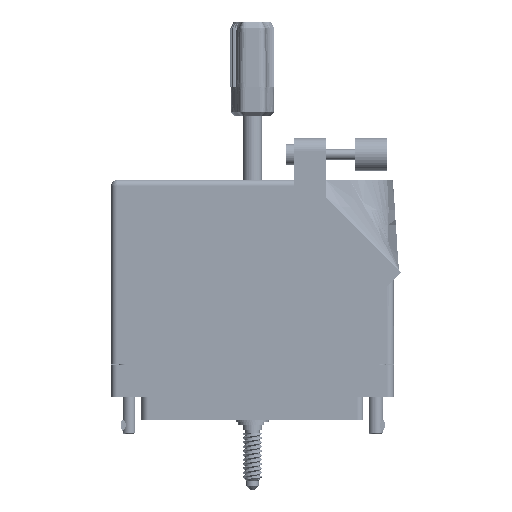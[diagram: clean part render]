
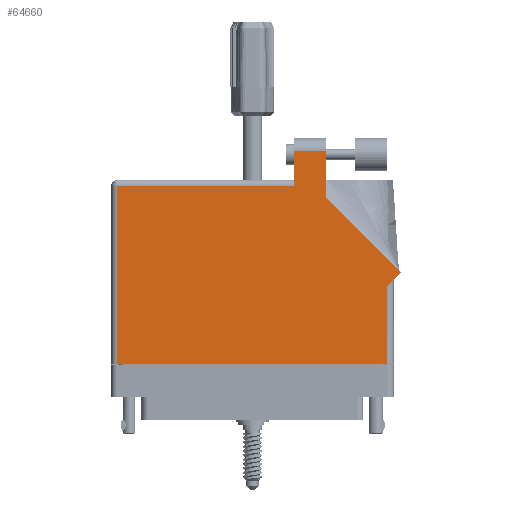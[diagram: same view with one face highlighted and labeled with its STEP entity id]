
A CAD part, front view. The second image highlights one B-rep face of the part: STEP entity #64660.
In plain terms, the highlighted face is planar.
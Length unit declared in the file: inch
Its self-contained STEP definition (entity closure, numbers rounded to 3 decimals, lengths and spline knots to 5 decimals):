
#67 = PLANE ( 'NONE',  #56658 ) ;
#3938 = VECTOR ( 'NONE', #38058, 39.37008 ) ;
#8568 = DIRECTION ( 'NONE',  ( 1., 0., 0. ) ) ;
#8986 = VERTEX_POINT ( 'NONE', #43268 ) ;
#9204 = CARTESIAN_POINT ( 'NONE',  ( 0.706, 1.50942, 0.617 ) ) ;
#10140 = EDGE_CURVE ( 'NONE', #48214, #16789, #78673, .T. ) ;
#13225 = DIRECTION ( 'NONE',  ( -1., 0., 0. ) ) ;
#14624 = CARTESIAN_POINT ( 'NONE',  ( 1.297, 0.653, 0.617 ) ) ;
#14733 = CARTESIAN_POINT ( 'NONE',  ( -1.359, 1.675, 0.617 ) ) ;
#14806 = LINE ( 'NONE', #53709, #89738 ) ;
#16759 = DIRECTION ( 'NONE',  ( -0.707, 0.707, 0. ) ) ;
#16789 = VERTEX_POINT ( 'NONE', #57808 ) ;
#18064 = ORIENTED_EDGE ( 'NONE', *, *, #82993, .T. ) ;
#18404 = LINE ( 'NONE', #21078, #95714 ) ;
#18605 = ORIENTED_EDGE ( 'NONE', *, *, #10140, .T. ) ;
#21078 = CARTESIAN_POINT ( 'NONE',  ( 0.399, 1.95, 0.617 ) ) ;
#22738 = EDGE_CURVE ( 'NONE', #31635, #35721, #92429, .T. ) ;
#23988 = ORIENTED_EDGE ( 'NONE', *, *, #61088, .T. ) ;
#24081 = EDGE_CURVE ( 'NONE', #64837, #48214, #18404, .T. ) ;
#28603 = VERTEX_POINT ( 'NONE', #34846 ) ;
#31635 = VERTEX_POINT ( 'NONE', #86220 ) ;
#34685 = ORIENTED_EDGE ( 'NONE', *, *, #24081, .T. ) ;
#34846 = CARTESIAN_POINT ( 'NONE',  ( 1.297, -0.1, 0.617 ) ) ;
#35706 = DIRECTION ( 'NONE',  ( 0., -1., 0. ) ) ;
#35721 = VERTEX_POINT ( 'NONE', #9204 ) ;
#37009 = DIRECTION ( 'NONE',  ( 0., 0., -1. ) ) ;
#38058 = DIRECTION ( 'NONE',  ( 0.707, 0.707, 0. ) ) ;
#39983 = EDGE_CURVE ( 'NONE', #16789, #8986, #71394, .T. ) ;
#43081 = EDGE_CURVE ( 'NONE', #28603, #45886, #14806, .T. ) ;
#43268 = CARTESIAN_POINT ( 'NONE',  ( -1.297, 1.613, 0.617 ) ) ;
#43524 = VECTOR ( 'NONE', #72002, 39.37008 ) ;
#44929 = ORIENTED_EDGE ( 'NONE', *, *, #22738, .T. ) ;
#45886 = VERTEX_POINT ( 'NONE', #14624 ) ;
#47236 = CARTESIAN_POINT ( 'NONE',  ( 1.42971, 0.78571, 0.617 ) ) ;
#48214 = VERTEX_POINT ( 'NONE', #66059 ) ;
#49573 = LINE ( 'NONE', #72078, #87015 ) ;
#49767 = DIRECTION ( 'NONE',  ( 0., -1., 0. ) ) ;
#50026 = CARTESIAN_POINT ( 'NONE',  ( 0.706, 1.50942, 0.617 ) ) ;
#53709 = CARTESIAN_POINT ( 'NONE',  ( 1.297, 0.715, 0.617 ) ) ;
#54650 = EDGE_CURVE ( 'NONE', #35721, #64837, #92772, .T. ) ;
#55277 = VECTOR ( 'NONE', #87617, 39.37008 ) ;
#56055 = VECTOR ( 'NONE', #16759, 39.37008 ) ;
#56318 = VERTEX_POINT ( 'NONE', #95928 ) ;
#56363 = VECTOR ( 'NONE', #49767, 39.37008 ) ;
#56658 = AXIS2_PLACEMENT_3D ( 'NONE', #14733, #37009, #75305 ) ;
#57808 = CARTESIAN_POINT ( 'NONE',  ( 0.399, 1.613, 0.617 ) ) ;
#61088 = EDGE_CURVE ( 'NONE', #56318, #28603, #96309, .T. ) ;
#63380 = CARTESIAN_POINT ( 'NONE',  ( -1.359, 1.613, 0.617 ) ) ;
#64660 = ADVANCED_FACE ( 'NONE', ( #74551 ), #67, .F. ) ;
#64837 = VERTEX_POINT ( 'NONE', #83460 ) ;
#66059 = CARTESIAN_POINT ( 'NONE',  ( 0.399, 1.95, 0.617 ) ) ;
#67202 = EDGE_LOOP ( 'NONE', ( #75527, #34685, #18605, #90942, #95452, #23988, #86889, #18064, #44929 ) ) ;
#69805 = CARTESIAN_POINT ( 'NONE',  ( -1.359, -0.1, 0.617 ) ) ;
#71394 = LINE ( 'NONE', #63380, #43524 ) ;
#72002 = DIRECTION ( 'NONE',  ( -1., 0., 0. ) ) ;
#72078 = CARTESIAN_POINT ( 'NONE',  ( -1.297, -0.1, 0.617 ) ) ;
#74551 = FACE_OUTER_BOUND ( 'NONE', #67202, .T. ) ;
#75305 = DIRECTION ( 'NONE',  ( -1., 0., 0. ) ) ;
#75527 = ORIENTED_EDGE ( 'NONE', *, *, #54650, .T. ) ;
#78673 = LINE ( 'NONE', #87360, #56363 ) ;
#82830 = DIRECTION ( 'NONE',  ( 0., 1., 0. ) ) ;
#82993 = EDGE_CURVE ( 'NONE', #45886, #31635, #83562, .T. ) ;
#83460 = CARTESIAN_POINT ( 'NONE',  ( 0.706, 1.95, 0.617 ) ) ;
#83562 = LINE ( 'NONE', #90752, #3938 ) ;
#86220 = CARTESIAN_POINT ( 'NONE',  ( 1.42971, 0.78571, 0.617 ) ) ;
#86889 = ORIENTED_EDGE ( 'NONE', *, *, #43081, .T. ) ;
#87015 = VECTOR ( 'NONE', #35706, 39.37008 ) ;
#87360 = CARTESIAN_POINT ( 'NONE',  ( 0.399, 1.675, 0.617 ) ) ;
#87617 = DIRECTION ( 'NONE',  ( 0., 1., 0. ) ) ;
#88022 = VECTOR ( 'NONE', #8568, 39.37008 ) ;
#89738 = VECTOR ( 'NONE', #82830, 39.37008 ) ;
#90752 = CARTESIAN_POINT ( 'NONE',  ( 1.359, 0.715, 0.617 ) ) ;
#90942 = ORIENTED_EDGE ( 'NONE', *, *, #39983, .T. ) ;
#91523 = EDGE_CURVE ( 'NONE', #8986, #56318, #49573, .T. ) ;
#92429 = LINE ( 'NONE', #47236, #56055 ) ;
#92772 = LINE ( 'NONE', #50026, #55277 ) ;
#95452 = ORIENTED_EDGE ( 'NONE', *, *, #91523, .T. ) ;
#95714 = VECTOR ( 'NONE', #13225, 39.37008 ) ;
#95928 = CARTESIAN_POINT ( 'NONE',  ( -1.297, -0.1, 0.617 ) ) ;
#96309 = LINE ( 'NONE', #69805, #88022 ) ;
